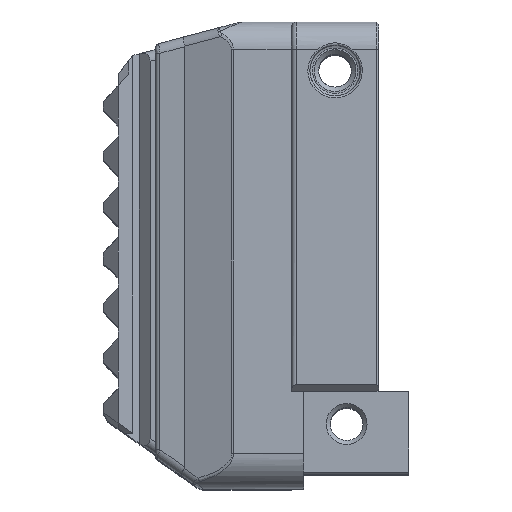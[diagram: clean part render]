
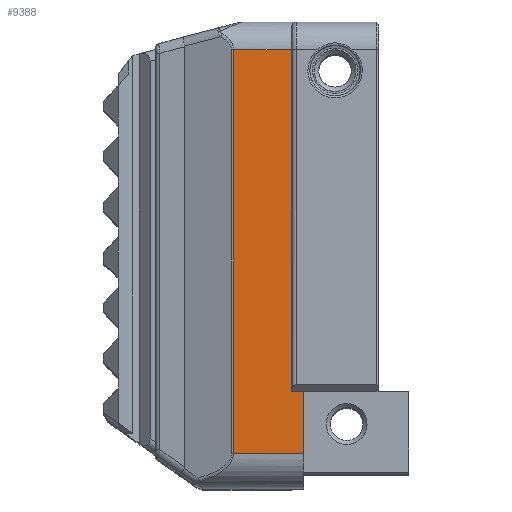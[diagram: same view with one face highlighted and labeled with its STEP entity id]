
A CAD part, top view. The second image highlights one B-rep face of the part: STEP entity #9388.
In plain terms, the highlighted planar face has unit normal (0, 0, 1).
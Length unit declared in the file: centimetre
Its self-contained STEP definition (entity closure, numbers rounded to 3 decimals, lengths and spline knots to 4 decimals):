
#764=LINE($,#17742,#1589);
#814=LINE($,#18270,#1639);
#815=LINE($,#18356,#1640);
#821=LINE($,#18471,#1646);
#822=LINE($,#18474,#1647);
#823=LINE($,#18475,#1648);
#1589=VECTOR($,#11839,6.7738);
#1639=VECTOR($,#11973,1.1508);
#1640=VECTOR($,#11988,8.0084);
#1646=VECTOR($,#12010,1.3908);
#1647=VECTOR($,#12013,0.24);
#1648=VECTOR($,#12014,1.2346);
#2201=PLANE($,#10167);
#2925=FACE_OUTER_BOUND($,#3563,.T.);
#3563=EDGE_LOOP($,(#7845,#7846,#7847,#7848,#7849,#7850));
#4573=VERTEX_POINT($,#17737);
#4574=VERTEX_POINT($,#17740);
#4610=VERTEX_POINT($,#18268);
#4616=VERTEX_POINT($,#18354);
#4626=VERTEX_POINT($,#18469);
#4627=VERTEX_POINT($,#18473);
#5681=EDGE_CURVE($,#4573,#4574,#764,.T.);
#5749=EDGE_CURVE($,#4610,#4574,#814,.T.);
#5759=EDGE_CURVE($,#4616,#4610,#815,.T.);
#5775=EDGE_CURVE($,#4616,#4626,#821,.T.);
#5776=EDGE_CURVE($,#4573,#4627,#822,.T.);
#5777=EDGE_CURVE($,#4626,#4627,#823,.T.);
#7845=ORIENTED_EDGE($,*,*,#5776,.F.);
#7846=ORIENTED_EDGE($,*,*,#5681,.T.);
#7847=ORIENTED_EDGE($,*,*,#5749,.F.);
#7848=ORIENTED_EDGE($,*,*,#5759,.F.);
#7849=ORIENTED_EDGE($,*,*,#5775,.T.);
#7850=ORIENTED_EDGE($,*,*,#5777,.T.);
#9388=ADVANCED_FACE($,(#2925),#2201,.T.);
#10167=AXIS2_PLACEMENT_3D($,#18472,#12011,#12012);
#11839=DIRECTION($,(0.,1.,0.));
#11973=DIRECTION($,(1.,0.,0.));
#11988=DIRECTION($,(0.,1.,0.));
#12010=DIRECTION($,(1.,0.,0.));
#12011=DIRECTION('center_axis',(0.,0.,
1.));
#12012=DIRECTION('ref_axis',(1.,0.,0.));
#12013=DIRECTION($,(1.,0.,0.));
#12014=DIRECTION($,(0.,1.,0.));
#17737=CARTESIAN_POINT('',(-19.5982,0.5867,11.9567));
#17740=CARTESIAN_POINT('',(-19.5982,7.3605,11.9567));
#17742=CARTESIAN_POINT($,(-19.5982,-0.4145,11.9567));
#18268=CARTESIAN_POINT('',(-20.749,7.3605,11.9567));
#18270=CARTESIAN_POINT($,(-21.3743,7.3605,11.9567));
#18354=CARTESIAN_POINT('',(-20.749,-0.6479,11.9567));
#18356=CARTESIAN_POINT($,(-20.749,-0.8841,11.9567));
#18469=CARTESIAN_POINT('',(-19.3582,-0.6479,11.9567));
#18471=CARTESIAN_POINT($,(-20.3968,-0.6479,11.9567));
#18472=CARTESIAN_POINT('Origin',(-20.3968,-0.4145,11.9567));
#18473=CARTESIAN_POINT('',(-19.3582,0.5867,11.9567));
#18474=CARTESIAN_POINT($,(-19.6325,0.5867,11.9567));
#18475=CARTESIAN_POINT($,(-19.3582,-0.4145,11.9567));
